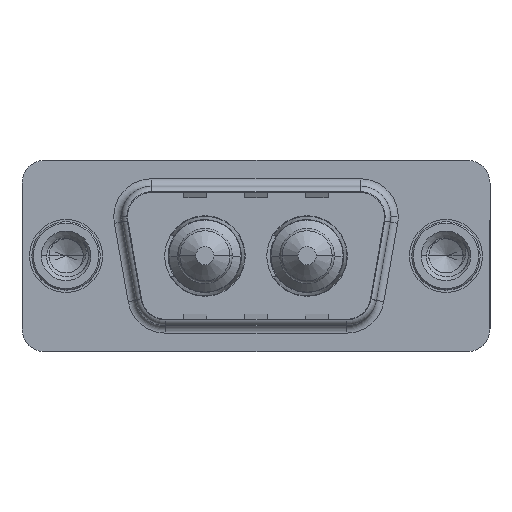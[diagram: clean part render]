
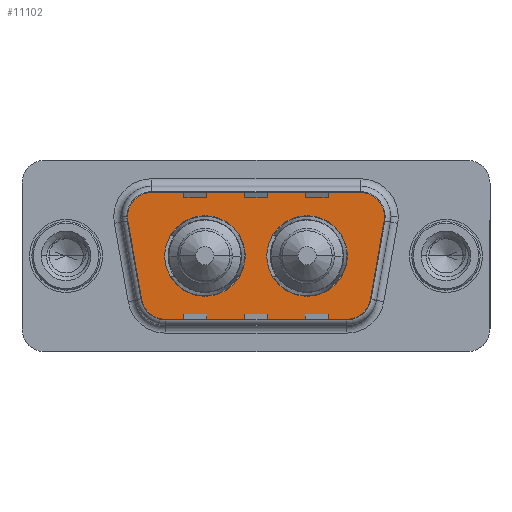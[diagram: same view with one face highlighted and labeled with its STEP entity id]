
A CAD part, top view. The second image highlights one B-rep face of the part: STEP entity #11102.
In plain terms, the highlighted planar face has unit normal (0, 0, 1).
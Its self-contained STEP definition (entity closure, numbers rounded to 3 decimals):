
#125 = DIRECTION ( 'NONE',  ( 0., 0., 1. ) ) ;
#155 = EDGE_CURVE ( 'NONE', #12240, #7677, #5706, .T. ) ;
#215 = VERTEX_POINT ( 'NONE', #2162 ) ;
#313 = ORIENTED_EDGE ( 'NONE', *, *, #155, .T. ) ;
#610 = FACE_OUTER_BOUND ( 'NONE', #7437, .T. ) ;
#660 = VERTEX_POINT ( 'NONE', #10533 ) ;
#874 = EDGE_CURVE ( 'NONE', #5546, #12240, #6817, .T. ) ;
#1026 = PLANE ( 'NONE',  #5497 ) ;
#1034 = CARTESIAN_POINT ( 'NONE',  ( 18.51, 0., 0. ) ) ;
#1045 = CARTESIAN_POINT ( 'NONE',  ( 21.534, 2.553, 0. ) ) ;
#1350 = ORIENTED_EDGE ( 'NONE', *, *, #2227, .T. ) ;
#1447 = CIRCLE ( 'NONE', #13357, 2.65 ) ;
#1739 = CIRCLE ( 'NONE', #6339, 2. ) ;
#1881 = ORIENTED_EDGE ( 'NONE', *, *, #9315, .T. ) ;
#2024 = CARTESIAN_POINT ( 'NONE',  ( 6.459, -2.9, 0. ) ) ;
#2082 = CARTESIAN_POINT ( 'NONE',  ( 3.466, 2.553, 0. ) ) ;
#2162 = CARTESIAN_POINT ( 'NONE',  ( 13.21, 0., 0. ) ) ;
#2227 = EDGE_CURVE ( 'NONE', #13274, #3068, #13102, .T. ) ;
#2354 = CIRCLE ( 'NONE', #7408, 2.65 ) ;
#2478 = DIRECTION ( 'NONE',  ( 1., 0., 0. ) ) ;
#2489 = EDGE_CURVE ( 'NONE', #7677, #3487, #13256, .T. ) ;
#2674 = VECTOR ( 'NONE', #8265, 1000. ) ;
#2844 = DIRECTION ( 'NONE',  ( 0., 0., 1. ) ) ;
#2984 = VERTEX_POINT ( 'NONE', #1034 ) ;
#3065 = DIRECTION ( 'NONE',  ( -1., 0., 0. ) ) ;
#3068 = VERTEX_POINT ( 'NONE', #8356 ) ;
#3360 = FACE_BOUND ( 'NONE', #5134, .T. ) ;
#3389 = CARTESIAN_POINT ( 'NONE',  ( 5.436, 4.9, 0. ) ) ;
#3401 = DIRECTION ( 'NONE',  ( 0., 0., 1. ) ) ;
#3487 = VERTEX_POINT ( 'NONE', #9985 ) ;
#3633 = CARTESIAN_POINT ( 'NONE',  ( 5.436, 4.9, 0. ) ) ;
#4070 = ORIENTED_EDGE ( 'NONE', *, *, #8530, .F. ) ;
#4120 = DIRECTION ( 'NONE',  ( 0.174, 0.985, 0. ) ) ;
#4146 = DIRECTION ( 'NONE',  ( 1., 0., 0. ) ) ;
#4170 = ORIENTED_EDGE ( 'NONE', *, *, #7529, .F. ) ;
#4263 = CARTESIAN_POINT ( 'NONE',  ( 18.541, -2.9, 0. ) ) ;
#4422 = VERTEX_POINT ( 'NONE', #11683 ) ;
#4428 = DIRECTION ( 'NONE',  ( -1., 0., 0. ) ) ;
#4443 = CARTESIAN_POINT ( 'NONE',  ( 15.86, 0., 0. ) ) ;
#4557 = EDGE_CURVE ( 'NONE', #215, #2984, #2354, .T. ) ;
#4575 = CARTESIAN_POINT ( 'NONE',  ( 5.436, 2.9, 0. ) ) ;
#4619 = VERTEX_POINT ( 'NONE', #5709 ) ;
#4664 = CARTESIAN_POINT ( 'NONE',  ( 20.511, -3.247, 0. ) ) ;
#4668 = DIRECTION ( 'NONE',  ( 0., 0., 1. ) ) ;
#4712 = DIRECTION ( 'NONE',  ( 1., 0., 0. ) ) ;
#4714 = ORIENTED_EDGE ( 'NONE', *, *, #9634, .F. ) ;
#4978 = VECTOR ( 'NONE', #4120, 1000. ) ;
#5134 = EDGE_LOOP ( 'NONE', ( #4170, #5612 ) ) ;
#5306 = DIRECTION ( 'NONE',  ( 0., 0., 1. ) ) ;
#5456 = AXIS2_PLACEMENT_3D ( 'NONE', #9062, #2844, #10095 ) ;
#5479 = DIRECTION ( 'NONE',  ( 1., 0., 0. ) ) ;
#5497 = AXIS2_PLACEMENT_3D ( 'NONE', #6176, #10365, #4146 ) ;
#5546 = VERTEX_POINT ( 'NONE', #9046 ) ;
#5612 = ORIENTED_EDGE ( 'NONE', *, *, #4557, .F. ) ;
#5621 = CARTESIAN_POINT ( 'NONE',  ( 15.86, 0., 0. ) ) ;
#5662 = DIRECTION ( 'NONE',  ( 1., 0., 0. ) ) ;
#5706 = CIRCLE ( 'NONE', #11064, 2. ) ;
#5709 = CARTESIAN_POINT ( 'NONE',  ( 6.49, 0., 0. ) ) ;
#5974 = VECTOR ( 'NONE', #4428, 1000. ) ;
#5987 = CIRCLE ( 'NONE', #13015, 2.65 ) ;
#6056 = CARTESIAN_POINT ( 'NONE',  ( 19.564, 2.9, 0. ) ) ;
#6060 = CARTESIAN_POINT ( 'NONE',  ( 18.541, -4.9, 0. ) ) ;
#6176 = CARTESIAN_POINT ( 'NONE',  ( 18.541, -2.9, 0. ) ) ;
#6303 = LINE ( 'NONE', #3389, #5974 ) ;
#6331 = ORIENTED_EDGE ( 'NONE', *, *, #874, .T. ) ;
#6339 = AXIS2_PLACEMENT_3D ( 'NONE', #6056, #13323, #7104 ) ;
#6656 = DIRECTION ( 'NONE',  ( 1., 0., 0. ) ) ;
#6817 = LINE ( 'NONE', #9979, #9297 ) ;
#7104 = DIRECTION ( 'NONE',  ( -1., 0., 0. ) ) ;
#7408 = AXIS2_PLACEMENT_3D ( 'NONE', #5621, #12884, #6656 ) ;
#7437 = EDGE_LOOP ( 'NONE', ( #313, #12078, #9930, #8313, #1881, #1350, #8501, #10963, #6331 ) ) ;
#7529 = EDGE_CURVE ( 'NONE', #2984, #215, #1447, .T. ) ;
#7557 = CIRCLE ( 'NONE', #13159, 2. ) ;
#7677 = VERTEX_POINT ( 'NONE', #4664 ) ;
#8144 = AXIS2_PLACEMENT_3D ( 'NONE', #2024, #9280, #3065 ) ;
#8265 = DIRECTION ( 'NONE',  ( 0.174, -0.985, 0. ) ) ;
#8313 = ORIENTED_EDGE ( 'NONE', *, *, #10358, .T. ) ;
#8356 = CARTESIAN_POINT ( 'NONE',  ( 3.466, 2.553, 0. ) ) ;
#8447 = EDGE_CURVE ( 'NONE', #660, #5546, #9410, .T. ) ;
#8501 = ORIENTED_EDGE ( 'NONE', *, *, #12908, .T. ) ;
#8530 = EDGE_CURVE ( 'NONE', #12714, #4619, #5987, .T. ) ;
#8555 = CIRCLE ( 'NONE', #5456, 2.65 ) ;
#9046 = CARTESIAN_POINT ( 'NONE',  ( 6.459, -4.9, 0. ) ) ;
#9062 = CARTESIAN_POINT ( 'NONE',  ( 9.14, 0., 0. ) ) ;
#9280 = DIRECTION ( 'NONE',  ( 0., 0., 1. ) ) ;
#9297 = VECTOR ( 'NONE', #2478, 1000. ) ;
#9315 = EDGE_CURVE ( 'NONE', #11626, #13274, #6303, .T. ) ;
#9410 = CIRCLE ( 'NONE', #8144, 2. ) ;
#9624 = CARTESIAN_POINT ( 'NONE',  ( 19.564, 2.9, 0. ) ) ;
#9634 = EDGE_CURVE ( 'NONE', #4619, #12714, #8555, .T. ) ;
#9927 = AXIS2_PLACEMENT_3D ( 'NONE', #4575, #4668, #4712 ) ;
#9930 = ORIENTED_EDGE ( 'NONE', *, *, #11294, .T. ) ;
#9979 = CARTESIAN_POINT ( 'NONE',  ( 6.459, -4.9, 0. ) ) ;
#9985 = CARTESIAN_POINT ( 'NONE',  ( 21.534, 2.553, 0. ) ) ;
#10095 = DIRECTION ( 'NONE',  ( 1., 0., 0. ) ) ;
#10352 = EDGE_LOOP ( 'NONE', ( #4070, #4714 ) ) ;
#10358 = EDGE_CURVE ( 'NONE', #4422, #11626, #1739, .T. ) ;
#10365 = DIRECTION ( 'NONE',  ( 0., 0., 1. ) ) ;
#10533 = CARTESIAN_POINT ( 'NONE',  ( 4.489, -3.247, 0. ) ) ;
#10638 = LINE ( 'NONE', #2082, #2674 ) ;
#10684 = DIRECTION ( 'NONE',  ( -1., 0., 0. ) ) ;
#10962 = CARTESIAN_POINT ( 'NONE',  ( 11.79, 0., 0. ) ) ;
#10963 = ORIENTED_EDGE ( 'NONE', *, *, #8447, .T. ) ;
#11064 = AXIS2_PLACEMENT_3D ( 'NONE', #4263, #125, #5662 ) ;
#11102 = ADVANCED_FACE ( 'NONE', ( #3360, #11661, #610 ), #1026, .T. ) ;
#11294 = EDGE_CURVE ( 'NONE', #3487, #4422, #7557, .T. ) ;
#11549 = CARTESIAN_POINT ( 'NONE',  ( 9.14, 0., 0. ) ) ;
#11626 = VERTEX_POINT ( 'NONE', #12262 ) ;
#11661 = FACE_BOUND ( 'NONE', #10352, .T. ) ;
#11683 = CARTESIAN_POINT ( 'NONE',  ( 21.564, 2.9, 0. ) ) ;
#11719 = DIRECTION ( 'NONE',  ( 0., 0., 1. ) ) ;
#12078 = ORIENTED_EDGE ( 'NONE', *, *, #2489, .T. ) ;
#12240 = VERTEX_POINT ( 'NONE', #6060 ) ;
#12262 = CARTESIAN_POINT ( 'NONE',  ( 19.564, 4.9, 0. ) ) ;
#12575 = DIRECTION ( 'NONE',  ( 1., 0., 0. ) ) ;
#12714 = VERTEX_POINT ( 'NONE', #10962 ) ;
#12884 = DIRECTION ( 'NONE',  ( 0., 0., 1. ) ) ;
#12908 = EDGE_CURVE ( 'NONE', #3068, #660, #10638, .T. ) ;
#13015 = AXIS2_PLACEMENT_3D ( 'NONE', #11549, #5306, #12575 ) ;
#13102 = CIRCLE ( 'NONE', #9927, 2. ) ;
#13159 = AXIS2_PLACEMENT_3D ( 'NONE', #9624, #3401, #10684 ) ;
#13256 = LINE ( 'NONE', #1045, #4978 ) ;
#13274 = VERTEX_POINT ( 'NONE', #3633 ) ;
#13323 = DIRECTION ( 'NONE',  ( 0., 0., 1. ) ) ;
#13357 = AXIS2_PLACEMENT_3D ( 'NONE', #4443, #11719, #5479 ) ;
